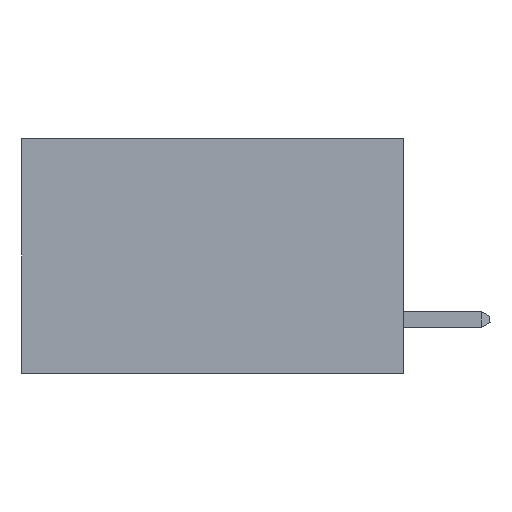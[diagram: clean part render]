
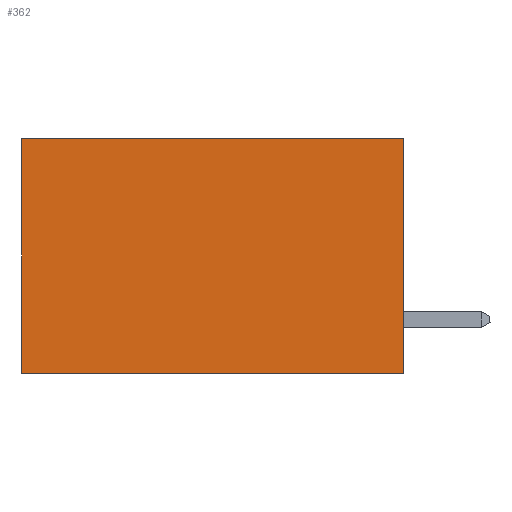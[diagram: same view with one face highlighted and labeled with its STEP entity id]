
A CAD part, left-side view. The second image highlights one B-rep face of the part: STEP entity #362.
In plain terms, the highlighted planar face has unit normal (-1, 0, 0).
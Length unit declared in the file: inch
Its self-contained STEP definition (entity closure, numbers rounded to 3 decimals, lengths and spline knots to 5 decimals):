
#148 = EDGE_CURVE ( 'NONE', #12535, #40874, #34914, .T. ) ;
#362 = ADVANCED_FACE ( 'NONE', ( #6691 ), #20571, .F. ) ;
#654 = LINE ( 'NONE', #8746, #38312 ) ;
#681 = CARTESIAN_POINT ( 'NONE',  ( 0.2875, 0., 0. ) ) ;
#831 = ORIENTED_EDGE ( 'NONE', *, *, #148, .T. ) ;
#3362 = LINE ( 'NONE', #10348, #16906 ) ;
#3405 = CARTESIAN_POINT ( 'NONE',  ( 0.2875, 0.6, -0.37 ) ) ;
#4055 = VERTEX_POINT ( 'NONE', #3405 ) ;
#4918 = DIRECTION ( 'NONE',  ( 0., 1., 0. ) ) ;
#5293 = VECTOR ( 'NONE', #13780, 39.37008 ) ;
#5647 = DIRECTION ( 'NONE',  ( 0., 0., -1. ) ) ;
#6691 = FACE_OUTER_BOUND ( 'NONE', #27889, .T. ) ;
#8746 = CARTESIAN_POINT ( 'NONE',  ( 0.2875, 0., 0. ) ) ;
#10338 = EDGE_CURVE ( 'NONE', #47920, #4055, #28158, .T. ) ;
#10348 = CARTESIAN_POINT ( 'NONE',  ( 0.2875, 0.6, 0. ) ) ;
#11285 = DIRECTION ( 'NONE',  ( 0., 0., -1. ) ) ;
#12535 = VERTEX_POINT ( 'NONE', #681 ) ;
#13780 = DIRECTION ( 'NONE',  ( 0., 1., 0. ) ) ;
#14752 = ORIENTED_EDGE ( 'NONE', *, *, #10338, .F. ) ;
#16906 = VECTOR ( 'NONE', #11285, 39.37008 ) ;
#17291 = CARTESIAN_POINT ( 'NONE',  ( 0.2875, 0., 0. ) ) ;
#18729 = EDGE_CURVE ( 'NONE', #12535, #47920, #654, .T. ) ;
#19632 = CARTESIAN_POINT ( 'NONE',  ( 0.2875, 0., -0.37 ) ) ;
#20571 = PLANE ( 'NONE',  #45430 ) ;
#23344 = DIRECTION ( 'NONE',  ( 0., 0., -1. ) ) ;
#27889 = EDGE_LOOP ( 'NONE', ( #30493, #14752, #40105, #831 ) ) ;
#28158 = LINE ( 'NONE', #38768, #5293 ) ;
#30493 = ORIENTED_EDGE ( 'NONE', *, *, #47721, .T. ) ;
#34914 = LINE ( 'NONE', #43100, #40828 ) ;
#38312 = VECTOR ( 'NONE', #23344, 39.37008 ) ;
#38768 = CARTESIAN_POINT ( 'NONE',  ( 0.2875, 0., -0.37 ) ) ;
#40105 = ORIENTED_EDGE ( 'NONE', *, *, #18729, .F. ) ;
#40828 = VECTOR ( 'NONE', #4918, 39.37008 ) ;
#40874 = VERTEX_POINT ( 'NONE', #46099 ) ;
#43100 = CARTESIAN_POINT ( 'NONE',  ( 0.2875, 0., 0. ) ) ;
#45430 = AXIS2_PLACEMENT_3D ( 'NONE', #17291, #46943, #5647 ) ;
#46099 = CARTESIAN_POINT ( 'NONE',  ( 0.2875, 0.6, 0. ) ) ;
#46943 = DIRECTION ( 'NONE',  ( 1., 0., 0. ) ) ;
#47721 = EDGE_CURVE ( 'NONE', #40874, #4055, #3362, .T. ) ;
#47920 = VERTEX_POINT ( 'NONE', #19632 ) ;
